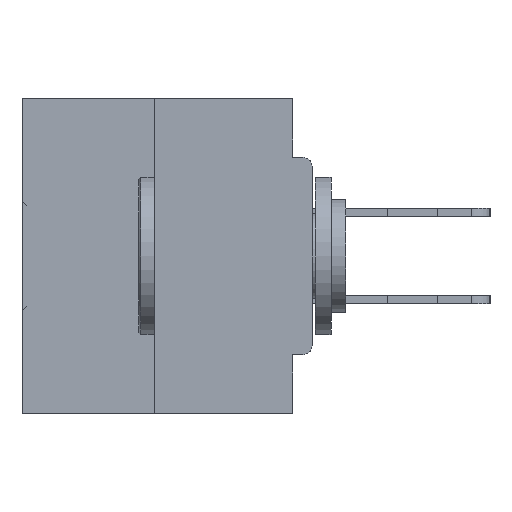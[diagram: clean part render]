
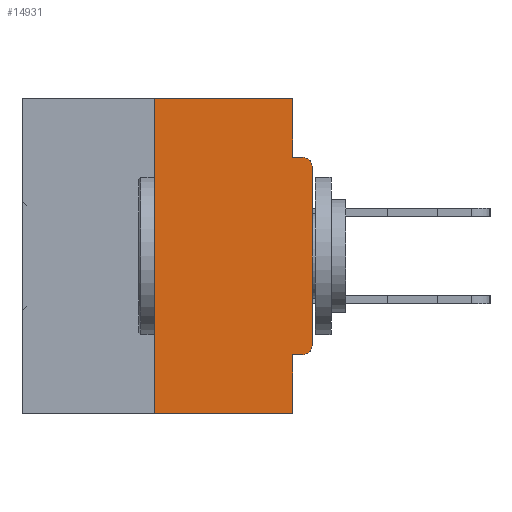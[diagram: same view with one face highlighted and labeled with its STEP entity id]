
A CAD part, left-side view. The second image highlights one B-rep face of the part: STEP entity #14931.
In plain terms, the highlighted planar face has unit normal (-1, 0, 0).
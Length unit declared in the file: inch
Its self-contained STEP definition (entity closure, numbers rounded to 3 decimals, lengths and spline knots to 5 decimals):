
#649 = ORIENTED_EDGE ( 'NONE', *, *, #37270, .F. ) ;
#947 = ORIENTED_EDGE ( 'NONE', *, *, #11298, .F. ) ;
#1247 = LINE ( 'NONE', #12769, #33861 ) ;
#3049 = VECTOR ( 'NONE', #31131, 39.37008 ) ;
#3642 = DIRECTION ( 'NONE',  ( 1., 0., 0. ) ) ;
#3810 = CARTESIAN_POINT ( 'NONE',  ( 0., 0., -0.1085 ) ) ;
#3942 = CARTESIAN_POINT ( 'NONE',  ( 0., 0.031, -0.5 ) ) ;
#6212 = EDGE_CURVE ( 'NONE', #34207, #35723, #1247, .T. ) ;
#6547 = DIRECTION ( 'NONE',  ( -1., 0., 0. ) ) ;
#6725 = ORIENTED_EDGE ( 'NONE', *, *, #23271, .F. ) ;
#7570 = DIRECTION ( 'NONE',  ( 0., 0., -1. ) ) ;
#7664 = EDGE_CURVE ( 'NONE', #19498, #34207, #14653, .T. ) ;
#8295 = AXIS2_PLACEMENT_3D ( 'NONE', #13614, #3642, #33991 ) ;
#8326 = CARTESIAN_POINT ( 'NONE',  ( 0., 0.031, -0.4065 ) ) ;
#8585 = DIRECTION ( 'NONE',  ( 0., -1., 0. ) ) ;
#9283 = AXIS2_PLACEMENT_3D ( 'NONE', #35063, #6547, #32053 ) ;
#9590 = EDGE_CURVE ( 'NONE', #35723, #26664, #21199, .T. ) ;
#10869 = VECTOR ( 'NONE', #24791, 39.37008 ) ;
#11093 = CARTESIAN_POINT ( 'NONE',  ( 0., 0.46, 0. ) ) ;
#11298 = EDGE_CURVE ( 'NONE', #17652, #26033, #15362, .T. ) ;
#12769 = CARTESIAN_POINT ( 'NONE',  ( 0., 0.031, 0. ) ) ;
#12949 = VECTOR ( 'NONE', #21939, 39.37008 ) ;
#13614 = CARTESIAN_POINT ( 'NONE',  ( 0., 0.46, 0. ) ) ;
#14245 = LINE ( 'NONE', #27974, #10869 ) ;
#14653 = LINE ( 'NONE', #11093, #12949 ) ;
#14931 = ADVANCED_FACE ( 'NONE', ( #24183 ), #20675, .F. ) ;
#15362 = LINE ( 'NONE', #32282, #24951 ) ;
#15490 = EDGE_CURVE ( 'NONE', #31076, #22368, #37116, .T. ) ;
#17071 = EDGE_CURVE ( 'NONE', #17652, #31076, #22261, .T. ) ;
#17321 = CARTESIAN_POINT ( 'NONE',  ( 0., 0.031, -0.0935 ) ) ;
#17652 = VERTEX_POINT ( 'NONE', #28651 ) ;
#17814 = DIRECTION ( 'NONE',  ( -1., 0., 0. ) ) ;
#19139 = DIRECTION ( 'NONE',  ( 0., 0., 1. ) ) ;
#19498 = VERTEX_POINT ( 'NONE', #32093 ) ;
#19584 = CARTESIAN_POINT ( 'NONE',  ( 0., 0., -0.0935 ) ) ;
#20222 = CIRCLE ( 'NONE', #44542, 0.015 ) ;
#20675 = PLANE ( 'NONE',  #8295 ) ;
#21199 = LINE ( 'NONE', #19584, #34762 ) ;
#21939 = DIRECTION ( 'NONE',  ( 0., -1., 0. ) ) ;
#22133 = LINE ( 'NONE', #27507, #3049 ) ;
#22240 = CARTESIAN_POINT ( 'NONE',  ( 0., 0.031, -0.5 ) ) ;
#22261 = CIRCLE ( 'NONE', #9283, 0.015 ) ;
#22368 = VERTEX_POINT ( 'NONE', #3810 ) ;
#22747 = VECTOR ( 'NONE', #7570, 39.37008 ) ;
#23271 = EDGE_CURVE ( 'NONE', #26033, #34911, #36892, .T. ) ;
#23342 = ORIENTED_EDGE ( 'NONE', *, *, #15490, .T. ) ;
#24183 = FACE_OUTER_BOUND ( 'NONE', #37053, .T. ) ;
#24574 = ORIENTED_EDGE ( 'NONE', *, *, #37406, .T. ) ;
#24758 = CARTESIAN_POINT ( 'NONE',  ( 0., 0., -0.3915 ) ) ;
#24791 = DIRECTION ( 'NONE',  ( 0., -1., 0. ) ) ;
#24951 = VECTOR ( 'NONE', #39608, 39.37008 ) ;
#26033 = VERTEX_POINT ( 'NONE', #8326 ) ;
#26664 = VERTEX_POINT ( 'NONE', #46177 ) ;
#27507 = CARTESIAN_POINT ( 'NONE',  ( 0., 0.25, 0. ) ) ;
#27526 = EDGE_CURVE ( 'NONE', #22368, #26664, #20222, .T. ) ;
#27974 = CARTESIAN_POINT ( 'NONE',  ( 0., 0.46, -0.5 ) ) ;
#28651 = CARTESIAN_POINT ( 'NONE',  ( 0., 0.015, -0.4065 ) ) ;
#29749 = ORIENTED_EDGE ( 'NONE', *, *, #17071, .T. ) ;
#31076 = VERTEX_POINT ( 'NONE', #24758 ) ;
#31131 = DIRECTION ( 'NONE',  ( 0., 0., 1. ) ) ;
#32053 = DIRECTION ( 'NONE',  ( 0., 0., -1. ) ) ;
#32077 = VECTOR ( 'NONE', #19139, 39.37008 ) ;
#32093 = CARTESIAN_POINT ( 'NONE',  ( 0., 0.25, 0. ) ) ;
#32282 = CARTESIAN_POINT ( 'NONE',  ( 0., 0., -0.4065 ) ) ;
#32366 = DIRECTION ( 'NONE',  ( 0., 0., -1. ) ) ;
#33802 = CARTESIAN_POINT ( 'NONE',  ( 0., 0., 0. ) ) ;
#33861 = VECTOR ( 'NONE', #41543, 39.37008 ) ;
#33991 = DIRECTION ( 'NONE',  ( 0., 0., -1. ) ) ;
#34207 = VERTEX_POINT ( 'NONE', #45855 ) ;
#34762 = VECTOR ( 'NONE', #8585, 39.37008 ) ;
#34911 = VERTEX_POINT ( 'NONE', #22240 ) ;
#35063 = CARTESIAN_POINT ( 'NONE',  ( 0., 0.015, -0.3915 ) ) ;
#35223 = ORIENTED_EDGE ( 'NONE', *, *, #27526, .T. ) ;
#35723 = VERTEX_POINT ( 'NONE', #17321 ) ;
#35993 = ORIENTED_EDGE ( 'NONE', *, *, #9590, .F. ) ;
#36892 = LINE ( 'NONE', #3942, #22747 ) ;
#37053 = EDGE_LOOP ( 'NONE', ( #39001, #649, #24574, #6725, #947, #29749, #23342, #35223, #35993, #40717 ) ) ;
#37116 = LINE ( 'NONE', #33802, #32077 ) ;
#37270 = EDGE_CURVE ( 'NONE', #39678, #19498, #22133, .T. ) ;
#37406 = EDGE_CURVE ( 'NONE', #39678, #34911, #14245, .T. ) ;
#39001 = ORIENTED_EDGE ( 'NONE', *, *, #7664, .F. ) ;
#39376 = CARTESIAN_POINT ( 'NONE',  ( 0., 0.015, -0.1085 ) ) ;
#39608 = DIRECTION ( 'NONE',  ( 0., 1., 0. ) ) ;
#39678 = VERTEX_POINT ( 'NONE', #46031 ) ;
#40717 = ORIENTED_EDGE ( 'NONE', *, *, #6212, .F. ) ;
#41543 = DIRECTION ( 'NONE',  ( 0., 0., -1. ) ) ;
#44542 = AXIS2_PLACEMENT_3D ( 'NONE', #39376, #17814, #32366 ) ;
#45855 = CARTESIAN_POINT ( 'NONE',  ( 0., 0.031, 0. ) ) ;
#46031 = CARTESIAN_POINT ( 'NONE',  ( 0., 0.25, -0.5 ) ) ;
#46177 = CARTESIAN_POINT ( 'NONE',  ( 0., 0.015, -0.0935 ) ) ;
